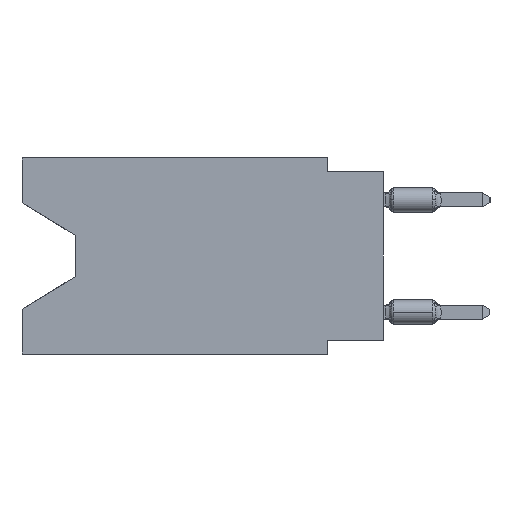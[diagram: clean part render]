
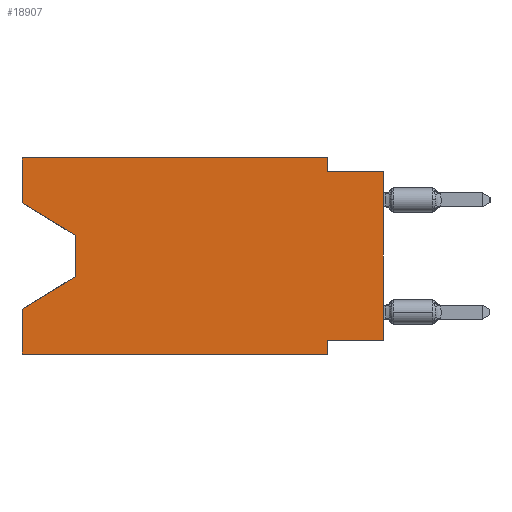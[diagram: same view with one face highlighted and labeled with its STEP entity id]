
A CAD part, left-side view. The second image highlights one B-rep face of the part: STEP entity #18907.
In plain terms, the highlighted planar face has unit normal (-1, 0, 0).
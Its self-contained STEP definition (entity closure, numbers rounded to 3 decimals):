
#127 = EDGE_CURVE ( 'NONE', #29573, #52548, #38130, .T. ) ;
#374 = EDGE_CURVE ( 'NONE', #9183, #24897, #43737, .T. ) ;
#435 = DIRECTION ( 'NONE',  ( 0., 0., 1. ) ) ;
#880 = ORIENTED_EDGE ( 'NONE', *, *, #892, .F. ) ;
#892 = EDGE_CURVE ( 'NONE', #3028, #9183, #36889, .T. ) ;
#913 = LINE ( 'NONE', #51816, #13770 ) ;
#982 = DIRECTION ( 'NONE',  ( 0., 0., -1. ) ) ;
#2203 = DIRECTION ( 'NONE',  ( 1., 0., 0. ) ) ;
#2339 = EDGE_CURVE ( 'NONE', #32549, #5426, #50927, .T. ) ;
#2411 = LINE ( 'NONE', #53879, #28876 ) ;
#3028 = VERTEX_POINT ( 'NONE', #16492 ) ;
#4369 = LINE ( 'NONE', #38703, #7507 ) ;
#5426 = VERTEX_POINT ( 'NONE', #15306 ) ;
#5712 = EDGE_CURVE ( 'NONE', #47845, #31597, #913, .T. ) ;
#7507 = VECTOR ( 'NONE', #435, 1000. ) ;
#7721 = ORIENTED_EDGE ( 'NONE', *, *, #50040, .T. ) ;
#7803 = EDGE_CURVE ( 'NONE', #32549, #29573, #2411, .T. ) ;
#8430 = ORIENTED_EDGE ( 'NONE', *, *, #127, .F. ) ;
#9183 = VERTEX_POINT ( 'NONE', #30735 ) ;
#9380 = VECTOR ( 'NONE', #35639, 1000. ) ;
#11571 = DIRECTION ( 'NONE',  ( 0., -1., 0. ) ) ;
#12528 = EDGE_CURVE ( 'NONE', #24897, #5426, #33299, .T. ) ;
#12585 = VERTEX_POINT ( 'NONE', #39188 ) ;
#13329 = ORIENTED_EDGE ( 'NONE', *, *, #374, .F. ) ;
#13770 = VECTOR ( 'NONE', #38901, 1000. ) ;
#14309 = CARTESIAN_POINT ( 'NONE',  ( 0., 16.383, -8.89 ) ) ;
#14624 = ORIENTED_EDGE ( 'NONE', *, *, #7803, .F. ) ;
#15219 = VECTOR ( 'NONE', #45678, 1000. ) ;
#15306 = CARTESIAN_POINT ( 'NONE',  ( 0., 0., -0.635 ) ) ;
#15879 = ORIENTED_EDGE ( 'NONE', *, *, #5712, .T. ) ;
#16333 = CARTESIAN_POINT ( 'NONE',  ( 0., 16.383, -6.852 ) ) ;
#16492 = CARTESIAN_POINT ( 'NONE',  ( 0., 16.383, 0. ) ) ;
#17546 = CARTESIAN_POINT ( 'NONE',  ( 0., 13.97, -5.385 ) ) ;
#18500 = LINE ( 'NONE', #27499, #9380 ) ;
#18907 = ADVANCED_FACE ( 'NONE', ( #41853 ), #23601, .F. ) ;
#19866 = VECTOR ( 'NONE', #982, 1000. ) ;
#20051 = ORIENTED_EDGE ( 'NONE', *, *, #42444, .F. ) ;
#21003 = CARTESIAN_POINT ( 'NONE',  ( 0., 13.97, -3.505 ) ) ;
#21547 = CARTESIAN_POINT ( 'NONE',  ( 0., 16.383, -2.038 ) ) ;
#22365 = CARTESIAN_POINT ( 'NONE',  ( 0., 2.54, 0. ) ) ;
#22835 = ORIENTED_EDGE ( 'NONE', *, *, #12528, .F. ) ;
#23261 = VECTOR ( 'NONE', #26465, 1000. ) ;
#23601 = PLANE ( 'NONE',  #35964 ) ;
#24032 = EDGE_CURVE ( 'NONE', #29795, #47845, #32512, .T. ) ;
#24897 = VERTEX_POINT ( 'NONE', #33483 ) ;
#25101 = ORIENTED_EDGE ( 'NONE', *, *, #2339, .T. ) ;
#25413 = CARTESIAN_POINT ( 'NONE',  ( 0., 0., -8.255 ) ) ;
#25814 = VECTOR ( 'NONE', #11571, 1000. ) ;
#26307 = DIRECTION ( 'NONE',  ( 0., 0., -1. ) ) ;
#26465 = DIRECTION ( 'NONE',  ( 0., 0., 1. ) ) ;
#26972 = LINE ( 'NONE', #14309, #34021 ) ;
#27028 = VECTOR ( 'NONE', #26307, 1000. ) ;
#27229 = CARTESIAN_POINT ( 'NONE',  ( 0., 2.54, -8.255 ) ) ;
#27499 = CARTESIAN_POINT ( 'NONE',  ( 0., 16.383, 0. ) ) ;
#28311 = VECTOR ( 'NONE', #46011, 1000. ) ;
#28633 = DIRECTION ( 'NONE',  ( 0., 0., -1. ) ) ;
#28876 = VECTOR ( 'NONE', #40693, 1000. ) ;
#29573 = VERTEX_POINT ( 'NONE', #27229 ) ;
#29795 = VERTEX_POINT ( 'NONE', #21003 ) ;
#30735 = CARTESIAN_POINT ( 'NONE',  ( 0., 2.54, 0. ) ) ;
#31104 = DIRECTION ( 'NONE',  ( 0., -0.855, -0.519 ) ) ;
#31597 = VERTEX_POINT ( 'NONE', #16333 ) ;
#31605 = CARTESIAN_POINT ( 'NONE',  ( 0., 2.54, -8.89 ) ) ;
#32512 = LINE ( 'NONE', #49669, #28311 ) ;
#32549 = VERTEX_POINT ( 'NONE', #25413 ) ;
#33299 = LINE ( 'NONE', #49893, #15219 ) ;
#33483 = CARTESIAN_POINT ( 'NONE',  ( 0., 2.54, -0.635 ) ) ;
#34021 = VECTOR ( 'NONE', #40181, 1000. ) ;
#34079 = ORIENTED_EDGE ( 'NONE', *, *, #39106, .F. ) ;
#35292 = EDGE_CURVE ( 'NONE', #55503, #29795, #39545, .T. ) ;
#35639 = DIRECTION ( 'NONE',  ( 0., 0., 1. ) ) ;
#35964 = AXIS2_PLACEMENT_3D ( 'NONE', #40751, #2203, #28633 ) ;
#36889 = LINE ( 'NONE', #54030, #25814 ) ;
#38130 = LINE ( 'NONE', #39242, #27028 ) ;
#38220 = VECTOR ( 'NONE', #31104, 1000. ) ;
#38703 = CARTESIAN_POINT ( 'NONE',  ( 0., 16.383, 0. ) ) ;
#38901 = DIRECTION ( 'NONE',  ( 0., 0.855, -0.519 ) ) ;
#39106 = EDGE_CURVE ( 'NONE', #55503, #3028, #4369, .T. ) ;
#39188 = CARTESIAN_POINT ( 'NONE',  ( 0., 16.383, -8.89 ) ) ;
#39242 = CARTESIAN_POINT ( 'NONE',  ( 0., 2.54, -8.89 ) ) ;
#39545 = LINE ( 'NONE', #45153, #38220 ) ;
#40181 = DIRECTION ( 'NONE',  ( 0., -1., 0. ) ) ;
#40693 = DIRECTION ( 'NONE',  ( 0., 1., 0. ) ) ;
#40751 = CARTESIAN_POINT ( 'NONE',  ( 0., 16.383, 0. ) ) ;
#41768 = ORIENTED_EDGE ( 'NONE', *, *, #35292, .T. ) ;
#41853 = FACE_OUTER_BOUND ( 'NONE', #49649, .T. ) ;
#42444 = EDGE_CURVE ( 'NONE', #12585, #31597, #18500, .T. ) ;
#43737 = LINE ( 'NONE', #22365, #19866 ) ;
#43897 = CARTESIAN_POINT ( 'NONE',  ( 0., 0., 0. ) ) ;
#45153 = CARTESIAN_POINT ( 'NONE',  ( 0., 16.383, -2.038 ) ) ;
#45678 = DIRECTION ( 'NONE',  ( 0., -1., 0. ) ) ;
#46011 = DIRECTION ( 'NONE',  ( 0., 0., -1. ) ) ;
#47845 = VERTEX_POINT ( 'NONE', #17546 ) ;
#49649 = EDGE_LOOP ( 'NONE', ( #41768, #53241, #15879, #20051, #7721, #8430, #14624, #25101, #22835, #13329, #880, #34079 ) ) ;
#49669 = CARTESIAN_POINT ( 'NONE',  ( 0., 13.97, -3.505 ) ) ;
#49893 = CARTESIAN_POINT ( 'NONE',  ( 0., 0., -0.635 ) ) ;
#50040 = EDGE_CURVE ( 'NONE', #12585, #52548, #26972, .T. ) ;
#50927 = LINE ( 'NONE', #43897, #23261 ) ;
#51816 = CARTESIAN_POINT ( 'NONE',  ( 0., 13.97, -5.385 ) ) ;
#52548 = VERTEX_POINT ( 'NONE', #31605 ) ;
#53241 = ORIENTED_EDGE ( 'NONE', *, *, #24032, .T. ) ;
#53879 = CARTESIAN_POINT ( 'NONE',  ( 0., 0., -8.255 ) ) ;
#54030 = CARTESIAN_POINT ( 'NONE',  ( 0., 16.383, 0. ) ) ;
#55503 = VERTEX_POINT ( 'NONE', #21547 ) ;
